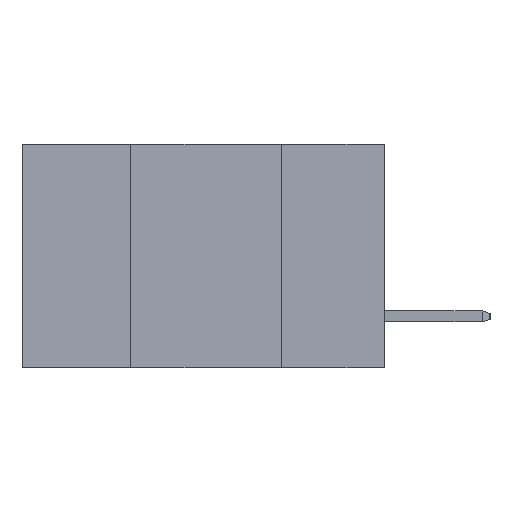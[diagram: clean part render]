
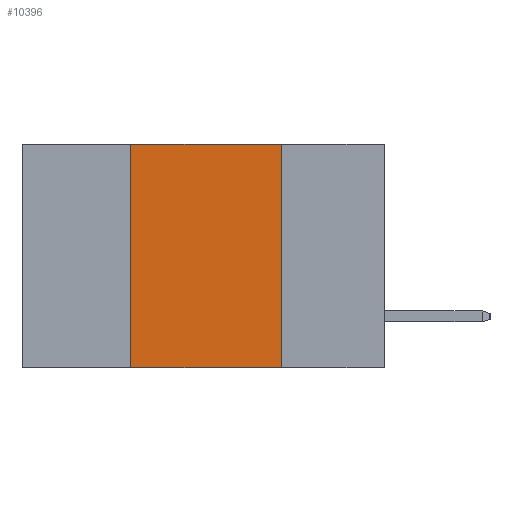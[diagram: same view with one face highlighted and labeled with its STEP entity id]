
A CAD part, left-side view. The second image highlights one B-rep face of the part: STEP entity #10396.
In plain terms, the highlighted planar face has unit normal (-1, 0, 0).
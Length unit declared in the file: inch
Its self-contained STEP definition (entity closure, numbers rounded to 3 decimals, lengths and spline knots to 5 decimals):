
#295 = VECTOR ( 'NONE', #1244, 39.37008 ) ;
#323 = VECTOR ( 'NONE', #5453, 39.37008 ) ;
#872 = VERTEX_POINT ( 'NONE', #5818 ) ;
#1244 = DIRECTION ( 'NONE',  ( 0., -1., 0. ) ) ;
#1644 = CARTESIAN_POINT ( 'NONE',  ( 0., 0.6, -0.37 ) ) ;
#2841 = ORIENTED_EDGE ( 'NONE', *, *, #10612, .T. ) ;
#2988 = VECTOR ( 'NONE', #10078, 39.37008 ) ;
#4280 = DIRECTION ( 'NONE',  ( 0., 0., 1. ) ) ;
#4901 = CARTESIAN_POINT ( 'NONE',  ( 0., 0.17, -0.37 ) ) ;
#5031 = CARTESIAN_POINT ( 'NONE',  ( 0., 0.17, -0.37 ) ) ;
#5074 = CARTESIAN_POINT ( 'NONE',  ( 0., 0.6, 0. ) ) ;
#5453 = DIRECTION ( 'NONE',  ( 0., -1., 0. ) ) ;
#5818 = CARTESIAN_POINT ( 'NONE',  ( 0., 0.42, -0.37 ) ) ;
#6140 = LINE ( 'NONE', #5031, #2988 ) ;
#7199 = DIRECTION ( 'NONE',  ( 1., 0., 0. ) ) ;
#7489 = CARTESIAN_POINT ( 'NONE',  ( 0., 0.17, 0. ) ) ;
#7761 = ORIENTED_EDGE ( 'NONE', *, *, #12561, .F. ) ;
#8067 = ORIENTED_EDGE ( 'NONE', *, *, #11905, .F. ) ;
#8555 = VERTEX_POINT ( 'NONE', #12132 ) ;
#9360 = VERTEX_POINT ( 'NONE', #4901 ) ;
#9423 = CARTESIAN_POINT ( 'NONE',  ( 0., 0.42, -0.37 ) ) ;
#9480 = VECTOR ( 'NONE', #4280, 39.37008 ) ;
#9491 = LINE ( 'NONE', #1644, #323 ) ;
#10078 = DIRECTION ( 'NONE',  ( 0., 0., -1. ) ) ;
#10211 = AXIS2_PLACEMENT_3D ( 'NONE', #5074, #7199, #14046 ) ;
#10302 = EDGE_LOOP ( 'NONE', ( #7761, #8067, #10696, #2841 ) ) ;
#10396 = ADVANCED_FACE ( 'NONE', ( #13602 ), #13093, .F. ) ;
#10612 = EDGE_CURVE ( 'NONE', #872, #9360, #9491, .T. ) ;
#10696 = ORIENTED_EDGE ( 'NONE', *, *, #11263, .F. ) ;
#11186 = CARTESIAN_POINT ( 'NONE',  ( 0., 0.6, 0. ) ) ;
#11263 = EDGE_CURVE ( 'NONE', #872, #8555, #12086, .T. ) ;
#11766 = LINE ( 'NONE', #11186, #295 ) ;
#11905 = EDGE_CURVE ( 'NONE', #8555, #12990, #11766, .T. ) ;
#12086 = LINE ( 'NONE', #9423, #9480 ) ;
#12132 = CARTESIAN_POINT ( 'NONE',  ( 0., 0.42, 0. ) ) ;
#12561 = EDGE_CURVE ( 'NONE', #12990, #9360, #6140, .T. ) ;
#12990 = VERTEX_POINT ( 'NONE', #7489 ) ;
#13093 = PLANE ( 'NONE',  #10211 ) ;
#13602 = FACE_OUTER_BOUND ( 'NONE', #10302, .T. ) ;
#14046 = DIRECTION ( 'NONE',  ( 0., 0., -1. ) ) ;
